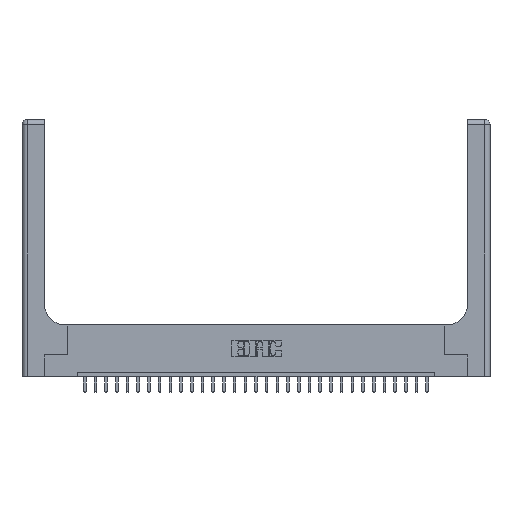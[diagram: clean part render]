
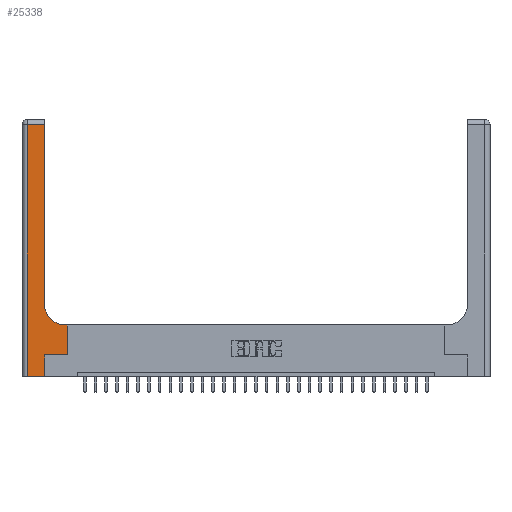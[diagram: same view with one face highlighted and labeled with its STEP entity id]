
A CAD part, top view. The second image highlights one B-rep face of the part: STEP entity #25338.
In plain terms, the highlighted planar face has unit normal (0, 0, 1).
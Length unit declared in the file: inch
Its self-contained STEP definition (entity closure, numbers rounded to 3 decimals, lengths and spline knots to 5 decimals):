
#65 = VERTEX_POINT ( 'NONE', #18940 ) ;
#79 = LINE ( 'NONE', #9340, #1884 ) ;
#106 = ORIENTED_EDGE ( 'NONE', *, *, #22442, .T. ) ;
#505 = LINE ( 'NONE', #783, #16122 ) ;
#783 = CARTESIAN_POINT ( 'NONE',  ( 0.26, 3., 0.37 ) ) ;
#1189 = DIRECTION ( 'NONE',  ( -1., 0., 0. ) ) ;
#1291 = VERTEX_POINT ( 'NONE', #16480 ) ;
#1884 = VECTOR ( 'NONE', #21313, 39.37008 ) ;
#2865 = VERTEX_POINT ( 'NONE', #13521 ) ;
#2878 = LINE ( 'NONE', #25759, #22454 ) ;
#2935 = VERTEX_POINT ( 'NONE', #15325 ) ;
#3147 = EDGE_CURVE ( 'NONE', #3880, #2865, #10065, .T. ) ;
#3269 = DIRECTION ( 'NONE',  ( -1., 0., 0. ) ) ;
#3347 = EDGE_CURVE ( 'NONE', #2935, #1291, #7118, .T. ) ;
#3880 = VERTEX_POINT ( 'NONE', #5005 ) ;
#4198 = ORIENTED_EDGE ( 'NONE', *, *, #3147, .T. ) ;
#4364 = EDGE_CURVE ( 'NONE', #2865, #65, #5495, .T. ) ;
#5005 = CARTESIAN_POINT ( 'NONE',  ( 0.26, 2.94, 0.37 ) ) ;
#5495 = LINE ( 'NONE', #20608, #12971 ) ;
#5850 = DIRECTION ( 'NONE',  ( 0., 1., 0. ) ) ;
#6075 = CARTESIAN_POINT ( 'NONE',  ( 0.528, 0.6, 0.37 ) ) ;
#6904 = DIRECTION ( 'NONE',  ( 0., 0., -1. ) ) ;
#7011 = DIRECTION ( 'NONE',  ( 1., 0., 0. ) ) ;
#7118 = LINE ( 'NONE', #17358, #21221 ) ;
#7511 = ORIENTED_EDGE ( 'NONE', *, *, #22864, .T. ) ;
#7853 = PLANE ( 'NONE',  #11867 ) ;
#8326 = ORIENTED_EDGE ( 'NONE', *, *, #10578, .T. ) ;
#8810 = VECTOR ( 'NONE', #5850, 39.37008 ) ;
#8926 = EDGE_CURVE ( 'NONE', #1291, #14378, #79, .T. ) ;
#9340 = CARTESIAN_POINT ( 'NONE',  ( 0.265, 0.25, 0.37 ) ) ;
#9541 = ORIENTED_EDGE ( 'NONE', *, *, #26697, .T. ) ;
#10065 = LINE ( 'NONE', #18245, #13706 ) ;
#10468 = AXIS2_PLACEMENT_3D ( 'NONE', #21211, #6904, #21474 ) ;
#10578 = EDGE_CURVE ( 'NONE', #20290, #3880, #505, .T. ) ;
#11112 = CARTESIAN_POINT ( 'NONE',  ( 0.528, 0.25, 0.37 ) ) ;
#11867 = AXIS2_PLACEMENT_3D ( 'NONE', #27127, #16428, #1189 ) ;
#12971 = VECTOR ( 'NONE', #16286, 39.37008 ) ;
#13016 = CARTESIAN_POINT ( 'NONE',  ( 0.26, 0.85, 0.37 ) ) ;
#13521 = CARTESIAN_POINT ( 'NONE',  ( 0.06, 2.94, 0.37 ) ) ;
#13706 = VECTOR ( 'NONE', #3269, 39.37008 ) ;
#13901 = ORIENTED_EDGE ( 'NONE', *, *, #8926, .T. ) ;
#14169 = LINE ( 'NONE', #20821, #8810 ) ;
#14378 = VERTEX_POINT ( 'NONE', #11112 ) ;
#14622 = EDGE_CURVE ( 'NONE', #26106, #20290, #23302, .T. ) ;
#15325 = CARTESIAN_POINT ( 'NONE',  ( 0.265, 0., 0.37 ) ) ;
#15642 = DIRECTION ( 'NONE',  ( -1., 0., 0. ) ) ;
#16122 = VECTOR ( 'NONE', #17695, 39.37008 ) ;
#16286 = DIRECTION ( 'NONE',  ( 0., -1., 0. ) ) ;
#16428 = DIRECTION ( 'NONE',  ( 0., 0., -1. ) ) ;
#16480 = CARTESIAN_POINT ( 'NONE',  ( 0.265, 0.25, 0.37 ) ) ;
#17353 = VERTEX_POINT ( 'NONE', #6075 ) ;
#17358 = CARTESIAN_POINT ( 'NONE',  ( 0.265, 0., 0.37 ) ) ;
#17650 = CARTESIAN_POINT ( 'NONE',  ( 0.51, 0.6, 0.37 ) ) ;
#17695 = DIRECTION ( 'NONE',  ( 0., 1., 0. ) ) ;
#17700 = ORIENTED_EDGE ( 'NONE', *, *, #3347, .T. ) ;
#18245 = CARTESIAN_POINT ( 'NONE',  ( 0., 2.94, 0.37 ) ) ;
#18864 = EDGE_LOOP ( 'NONE', ( #8326, #4198, #22338, #7511, #17700, #13901, #9541, #106, #23063 ) ) ;
#18940 = CARTESIAN_POINT ( 'NONE',  ( 0.06, 0., 0.37 ) ) ;
#19473 = DIRECTION ( 'NONE',  ( 0., 1., 0. ) ) ;
#19507 = CARTESIAN_POINT ( 'NONE',  ( 0., 0., 0.37 ) ) ;
#20290 = VERTEX_POINT ( 'NONE', #13016 ) ;
#20608 = CARTESIAN_POINT ( 'NONE',  ( 0.06, 3., 0.37 ) ) ;
#20821 = CARTESIAN_POINT ( 'NONE',  ( 0.528, 0.25, 0.37 ) ) ;
#21211 = CARTESIAN_POINT ( 'NONE',  ( 0.51, 0.85, 0.37 ) ) ;
#21221 = VECTOR ( 'NONE', #19473, 39.37008 ) ;
#21313 = DIRECTION ( 'NONE',  ( 1., 0., 0. ) ) ;
#21474 = DIRECTION ( 'NONE',  ( 1., 0., 0. ) ) ;
#21995 = LINE ( 'NONE', #19507, #22030 ) ;
#22030 = VECTOR ( 'NONE', #7011, 39.37008 ) ;
#22338 = ORIENTED_EDGE ( 'NONE', *, *, #4364, .T. ) ;
#22442 = EDGE_CURVE ( 'NONE', #17353, #26106, #2878, .T. ) ;
#22454 = VECTOR ( 'NONE', #15642, 39.37008 ) ;
#22864 = EDGE_CURVE ( 'NONE', #65, #2935, #21995, .T. ) ;
#23063 = ORIENTED_EDGE ( 'NONE', *, *, #14622, .T. ) ;
#23302 = CIRCLE ( 'NONE', #10468, 0.25 ) ;
#25338 = ADVANCED_FACE ( 'NONE', ( #26850 ), #7853, .F. ) ;
#25759 = CARTESIAN_POINT ( 'NONE',  ( 0.26, 0.6, 0.37 ) ) ;
#26106 = VERTEX_POINT ( 'NONE', #17650 ) ;
#26697 = EDGE_CURVE ( 'NONE', #14378, #17353, #14169, .T. ) ;
#26850 = FACE_OUTER_BOUND ( 'NONE', #18864, .T. ) ;
#27127 = CARTESIAN_POINT ( 'NONE',  ( 0., 3., 0.37 ) ) ;
